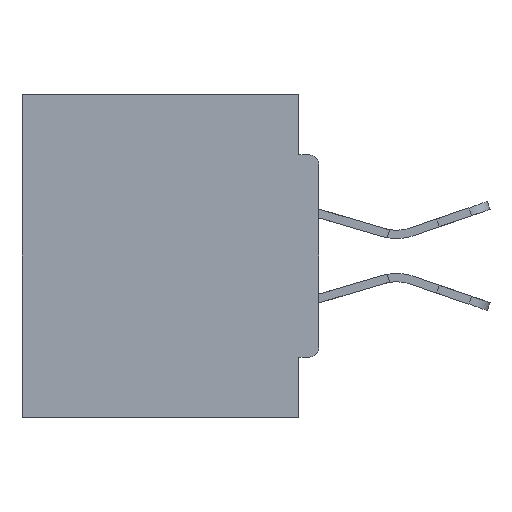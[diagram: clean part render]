
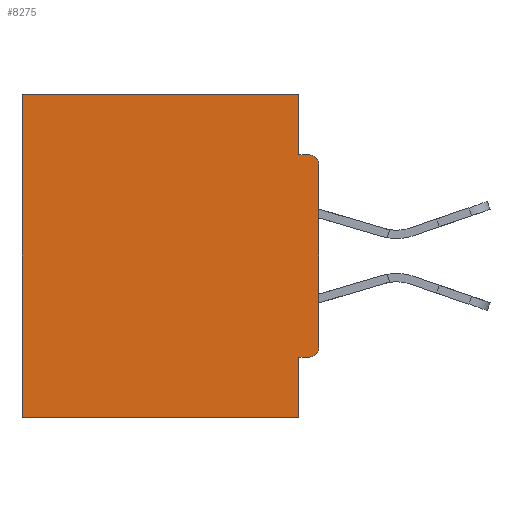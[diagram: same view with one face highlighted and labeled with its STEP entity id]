
A CAD part, left-side view. The second image highlights one B-rep face of the part: STEP entity #8275.
In plain terms, the highlighted planar face has unit normal (-1, 0, 0).
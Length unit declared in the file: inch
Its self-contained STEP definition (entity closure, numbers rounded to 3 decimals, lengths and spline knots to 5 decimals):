
#997 = DIRECTION ( 'NONE',  ( 1., 0., 0. ) ) ;
#1340 = EDGE_CURVE ( 'NONE', #3719, #4544, #13284, .T. ) ;
#1610 = EDGE_CURVE ( 'NONE', #19574, #9552, #37862, .T. ) ;
#2404 = VECTOR ( 'NONE', #18700, 39.37008 ) ;
#3131 = CARTESIAN_POINT ( 'NONE',  ( 0.298, 0., -0.0935 ) ) ;
#3719 = VERTEX_POINT ( 'NONE', #36252 ) ;
#4479 = AXIS2_PLACEMENT_3D ( 'NONE', #33675, #24644, #34068 ) ;
#4544 = VERTEX_POINT ( 'NONE', #22150 ) ;
#5216 = DIRECTION ( 'NONE',  ( 0., 0., -1. ) ) ;
#6108 = VERTEX_POINT ( 'NONE', #31164 ) ;
#7191 = VERTEX_POINT ( 'NONE', #7972 ) ;
#7607 = EDGE_CURVE ( 'NONE', #6108, #9552, #32576, .T. ) ;
#7705 = CARTESIAN_POINT ( 'NONE',  ( 0.298, 0., 0. ) ) ;
#7972 = CARTESIAN_POINT ( 'NONE',  ( 0.298, 0.031, -0.5 ) ) ;
#8248 = CARTESIAN_POINT ( 'NONE',  ( 0.298, 0., 0. ) ) ;
#8275 = ADVANCED_FACE ( 'NONE', ( #13485 ), #33985, .F. ) ;
#8418 = CARTESIAN_POINT ( 'NONE',  ( 0.298, 0., -0.1085 ) ) ;
#8502 = VERTEX_POINT ( 'NONE', #9717 ) ;
#8666 = CARTESIAN_POINT ( 'NONE',  ( 0.298, 0.46, 0. ) ) ;
#9088 = EDGE_CURVE ( 'NONE', #3719, #6108, #20962, .T. ) ;
#9402 = LINE ( 'NONE', #8666, #10335 ) ;
#9552 = VERTEX_POINT ( 'NONE', #36250 ) ;
#9717 = CARTESIAN_POINT ( 'NONE',  ( 0.298, 0.015, -0.4065 ) ) ;
#10293 = DIRECTION ( 'NONE',  ( 0., 0., -1. ) ) ;
#10335 = VECTOR ( 'NONE', #17767, 39.37008 ) ;
#11109 = DIRECTION ( 'NONE',  ( 0., 1., 0. ) ) ;
#11683 = VERTEX_POINT ( 'NONE', #27739 ) ;
#11775 = EDGE_LOOP ( 'NONE', ( #24033, #19749, #22312, #14311, #29196, #23635, #17737, #38155, #30647, #15165 ) ) ;
#11946 = EDGE_CURVE ( 'NONE', #8502, #13169, #24088, .T. ) ;
#12231 = VECTOR ( 'NONE', #15208, 39.37008 ) ;
#12681 = CIRCLE ( 'NONE', #32284, 0.015 ) ;
#12785 = EDGE_CURVE ( 'NONE', #8502, #11683, #12681, .T. ) ;
#12923 = CARTESIAN_POINT ( 'NONE',  ( 0.298, 0., -0.4065 ) ) ;
#13169 = VERTEX_POINT ( 'NONE', #22801 ) ;
#13284 = LINE ( 'NONE', #7705, #17022 ) ;
#13485 = FACE_OUTER_BOUND ( 'NONE', #11775, .T. ) ;
#14311 = ORIENTED_EDGE ( 'NONE', *, *, #1340, .T. ) ;
#14906 = DIRECTION ( 'NONE',  ( 0., 0., -1. ) ) ;
#15165 = ORIENTED_EDGE ( 'NONE', *, *, #21359, .F. ) ;
#15208 = DIRECTION ( 'NONE',  ( 0., -1., 0. ) ) ;
#15220 = EDGE_CURVE ( 'NONE', #4544, #28589, #9402, .T. ) ;
#16470 = AXIS2_PLACEMENT_3D ( 'NONE', #19284, #997, #10293 ) ;
#17022 = VECTOR ( 'NONE', #37979, 39.37008 ) ;
#17737 = ORIENTED_EDGE ( 'NONE', *, *, #18808, .F. ) ;
#17767 = DIRECTION ( 'NONE',  ( 0., 0., -1. ) ) ;
#18700 = DIRECTION ( 'NONE',  ( 0., 1., 0. ) ) ;
#18808 = EDGE_CURVE ( 'NONE', #13169, #7191, #36067, .T. ) ;
#19284 = CARTESIAN_POINT ( 'NONE',  ( 0.298, 0., 0. ) ) ;
#19556 = DIRECTION ( 'NONE',  ( 0., 0., -1. ) ) ;
#19574 = VERTEX_POINT ( 'NONE', #8418 ) ;
#19749 = ORIENTED_EDGE ( 'NONE', *, *, #7607, .F. ) ;
#20962 = LINE ( 'NONE', #22609, #28527 ) ;
#21359 = EDGE_CURVE ( 'NONE', #19574, #11683, #22885, .T. ) ;
#22150 = CARTESIAN_POINT ( 'NONE',  ( 0.298, 0.46, 0. ) ) ;
#22312 = ORIENTED_EDGE ( 'NONE', *, *, #9088, .F. ) ;
#22609 = CARTESIAN_POINT ( 'NONE',  ( 0.298, 0.031, -0.5 ) ) ;
#22801 = CARTESIAN_POINT ( 'NONE',  ( 0.298, 0.031, -0.4065 ) ) ;
#22885 = LINE ( 'NONE', #8248, #23326 ) ;
#23326 = VECTOR ( 'NONE', #38001, 39.37008 ) ;
#23635 = ORIENTED_EDGE ( 'NONE', *, *, #23841, .F. ) ;
#23841 = EDGE_CURVE ( 'NONE', #7191, #28589, #34146, .T. ) ;
#24033 = ORIENTED_EDGE ( 'NONE', *, *, #1610, .T. ) ;
#24088 = LINE ( 'NONE', #12923, #2404 ) ;
#24644 = DIRECTION ( 'NONE',  ( -1., 0., 0. ) ) ;
#26031 = VECTOR ( 'NONE', #11109, 39.37008 ) ;
#27064 = VECTOR ( 'NONE', #14906, 39.37008 ) ;
#27739 = CARTESIAN_POINT ( 'NONE',  ( 0.298, 0., -0.3915 ) ) ;
#28527 = VECTOR ( 'NONE', #19556, 39.37008 ) ;
#28589 = VERTEX_POINT ( 'NONE', #33561 ) ;
#29196 = ORIENTED_EDGE ( 'NONE', *, *, #15220, .T. ) ;
#30647 = ORIENTED_EDGE ( 'NONE', *, *, #12785, .T. ) ;
#31164 = CARTESIAN_POINT ( 'NONE',  ( 0.298, 0.031, -0.0935 ) ) ;
#32284 = AXIS2_PLACEMENT_3D ( 'NONE', #38364, #35605, #5216 ) ;
#32576 = LINE ( 'NONE', #3131, #12231 ) ;
#33033 = CARTESIAN_POINT ( 'NONE',  ( 0.298, 0.031, -0.5 ) ) ;
#33561 = CARTESIAN_POINT ( 'NONE',  ( 0.298, 0.46, -0.5 ) ) ;
#33675 = CARTESIAN_POINT ( 'NONE',  ( 0.298, 0.015, -0.1085 ) ) ;
#33985 = PLANE ( 'NONE',  #16470 ) ;
#34068 = DIRECTION ( 'NONE',  ( 0., 0., -1. ) ) ;
#34146 = LINE ( 'NONE', #38586, #26031 ) ;
#35605 = DIRECTION ( 'NONE',  ( -1., 0., 0. ) ) ;
#36067 = LINE ( 'NONE', #33033, #27064 ) ;
#36250 = CARTESIAN_POINT ( 'NONE',  ( 0.298, 0.015, -0.0935 ) ) ;
#36252 = CARTESIAN_POINT ( 'NONE',  ( 0.298, 0.031, 0. ) ) ;
#37862 = CIRCLE ( 'NONE', #4479, 0.015 ) ;
#37979 = DIRECTION ( 'NONE',  ( 0., 1., 0. ) ) ;
#38001 = DIRECTION ( 'NONE',  ( 0., 0., -1. ) ) ;
#38155 = ORIENTED_EDGE ( 'NONE', *, *, #11946, .F. ) ;
#38364 = CARTESIAN_POINT ( 'NONE',  ( 0.298, 0.015, -0.3915 ) ) ;
#38586 = CARTESIAN_POINT ( 'NONE',  ( 0.298, 0., -0.5 ) ) ;
